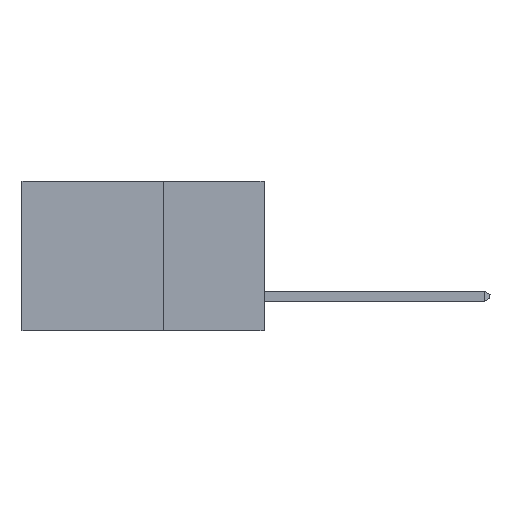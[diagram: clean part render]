
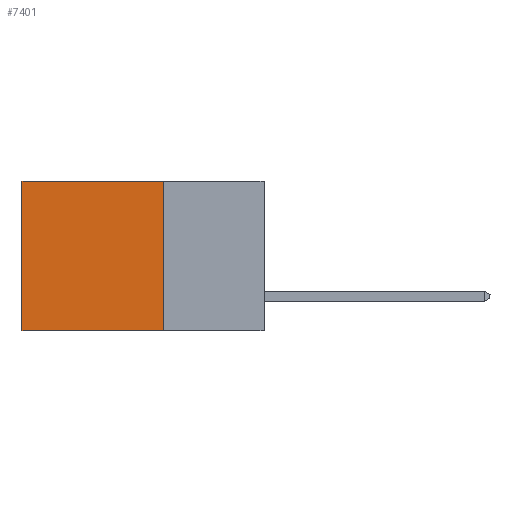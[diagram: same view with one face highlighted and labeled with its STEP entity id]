
A CAD part, left-side view. The second image highlights one B-rep face of the part: STEP entity #7401.
In plain terms, the highlighted planar face has unit normal (-1, 0, 0).
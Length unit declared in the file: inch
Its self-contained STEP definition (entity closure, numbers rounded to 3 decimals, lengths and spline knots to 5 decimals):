
#2220 = VECTOR ( 'NONE', #26073, 39.37008 ) ;
#2594 = EDGE_CURVE ( 'NONE', #22942, #13658, #10887, .T. ) ;
#6649 = VECTOR ( 'NONE', #26206, 39.37008 ) ;
#7401 = ADVANCED_FACE ( 'NONE', ( #14319 ), #8524, .F. ) ;
#7755 = VERTEX_POINT ( 'NONE', #14433 ) ;
#7922 = VECTOR ( 'NONE', #27162, 39.37008 ) ;
#8197 = VERTEX_POINT ( 'NONE', #19415 ) ;
#8441 = DIRECTION ( 'NONE',  ( 0., 0., -1. ) ) ;
#8524 = PLANE ( 'NONE',  #13770 ) ;
#10887 = LINE ( 'NONE', #13095, #6649 ) ;
#11060 = LINE ( 'NONE', #12389, #2220 ) ;
#12112 = VECTOR ( 'NONE', #20162, 39.37008 ) ;
#12389 = CARTESIAN_POINT ( 'NONE',  ( 0.298, 0.6, 0. ) ) ;
#13095 = CARTESIAN_POINT ( 'NONE',  ( 0.298, 0.25, 0. ) ) ;
#13164 = LINE ( 'NONE', #13610, #12112 ) ;
#13174 = ORIENTED_EDGE ( 'NONE', *, *, #15163, .T. ) ;
#13610 = CARTESIAN_POINT ( 'NONE',  ( 0.298, 0.25, -0.37 ) ) ;
#13658 = VERTEX_POINT ( 'NONE', #28993 ) ;
#13770 = AXIS2_PLACEMENT_3D ( 'NONE', #26426, #21937, #8441 ) ;
#14073 = ORIENTED_EDGE ( 'NONE', *, *, #26162, .T. ) ;
#14319 = FACE_OUTER_BOUND ( 'NONE', #22123, .T. ) ;
#14433 = CARTESIAN_POINT ( 'NONE',  ( 0.298, 0.6, 0. ) ) ;
#14744 = EDGE_CURVE ( 'NONE', #13658, #8197, #13164, .T. ) ;
#15163 = EDGE_CURVE ( 'NONE', #7755, #8197, #11060, .T. ) ;
#19415 = CARTESIAN_POINT ( 'NONE',  ( 0.298, 0.6, -0.37 ) ) ;
#20162 = DIRECTION ( 'NONE',  ( 0., 1., 0. ) ) ;
#21937 = DIRECTION ( 'NONE',  ( 1., 0., 0. ) ) ;
#22123 = EDGE_LOOP ( 'NONE', ( #13174, #28362, #28250, #14073 ) ) ;
#22942 = VERTEX_POINT ( 'NONE', #22996 ) ;
#22996 = CARTESIAN_POINT ( 'NONE',  ( 0.298, 0.25, 0. ) ) ;
#26073 = DIRECTION ( 'NONE',  ( 0., 0., -1. ) ) ;
#26162 = EDGE_CURVE ( 'NONE', #22942, #7755, #27401, .T. ) ;
#26206 = DIRECTION ( 'NONE',  ( 0., 0., -1. ) ) ;
#26426 = CARTESIAN_POINT ( 'NONE',  ( 0.298, 0.25, 0. ) ) ;
#27046 = CARTESIAN_POINT ( 'NONE',  ( 0.298, 0.25, 0. ) ) ;
#27162 = DIRECTION ( 'NONE',  ( 0., 1., 0. ) ) ;
#27401 = LINE ( 'NONE', #27046, #7922 ) ;
#28250 = ORIENTED_EDGE ( 'NONE', *, *, #2594, .F. ) ;
#28362 = ORIENTED_EDGE ( 'NONE', *, *, #14744, .F. ) ;
#28993 = CARTESIAN_POINT ( 'NONE',  ( 0.298, 0.25, -0.37 ) ) ;
